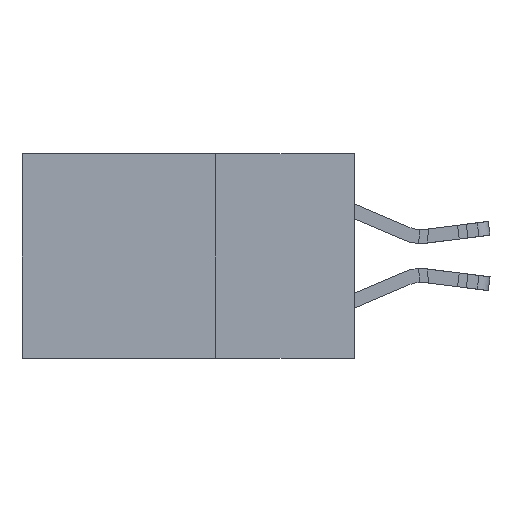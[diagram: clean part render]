
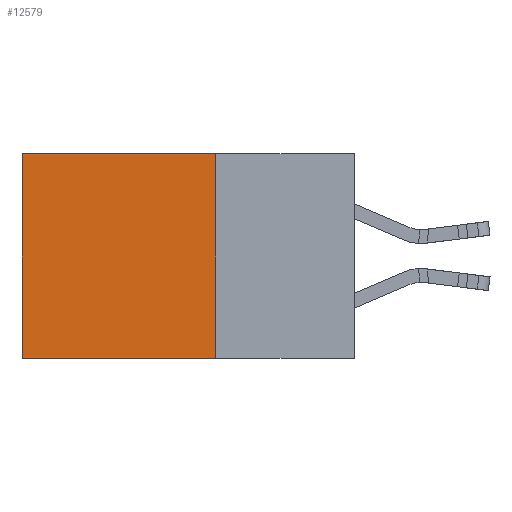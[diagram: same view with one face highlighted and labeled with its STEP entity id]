
A CAD part, left-side view. The second image highlights one B-rep face of the part: STEP entity #12579.
In plain terms, the highlighted planar face has unit normal (-1, 0, 0).
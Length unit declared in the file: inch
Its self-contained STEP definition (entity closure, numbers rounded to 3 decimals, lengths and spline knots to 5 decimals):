
#718 = VERTEX_POINT ( 'NONE', #25084 ) ;
#1443 = VECTOR ( 'NONE', #6467, 39.37008 ) ;
#3622 = EDGE_LOOP ( 'NONE', ( #19263, #14002, #20870, #13499 ) ) ;
#3845 = VERTEX_POINT ( 'NONE', #14104 ) ;
#5294 = EDGE_CURVE ( 'NONE', #3845, #718, #21139, .T. ) ;
#5967 = CARTESIAN_POINT ( 'NONE',  ( 0.2615, 0.25, 0. ) ) ;
#6199 = VECTOR ( 'NONE', #9591, 39.37008 ) ;
#6421 = CARTESIAN_POINT ( 'NONE',  ( 0.2615, 0.25, -0.37 ) ) ;
#6467 = DIRECTION ( 'NONE',  ( 0., 0., -1. ) ) ;
#7890 = PLANE ( 'NONE',  #24392 ) ;
#7988 = DIRECTION ( 'NONE',  ( 0., 1., 0. ) ) ;
#9591 = DIRECTION ( 'NONE',  ( 0., 1., 0. ) ) ;
#9822 = CARTESIAN_POINT ( 'NONE',  ( 0.2615, 0.25, -0.37 ) ) ;
#9906 = DIRECTION ( 'NONE',  ( 0., 0., -1. ) ) ;
#10601 = VECTOR ( 'NONE', #24249, 39.37008 ) ;
#10788 = EDGE_CURVE ( 'NONE', #19904, #14408, #12145, .T. ) ;
#11529 = LINE ( 'NONE', #23343, #6199 ) ;
#12145 = LINE ( 'NONE', #22352, #1443 ) ;
#12579 = ADVANCED_FACE ( 'NONE', ( #23174 ), #7890, .F. ) ;
#13499 = ORIENTED_EDGE ( 'NONE', *, *, #24561, .T. ) ;
#13743 = LINE ( 'NONE', #5967, #14381 ) ;
#14002 = ORIENTED_EDGE ( 'NONE', *, *, #17277, .F. ) ;
#14104 = CARTESIAN_POINT ( 'NONE',  ( 0.2615, 0.25, 0. ) ) ;
#14381 = VECTOR ( 'NONE', #7988, 39.37008 ) ;
#14408 = VERTEX_POINT ( 'NONE', #22714 ) ;
#17277 = EDGE_CURVE ( 'NONE', #718, #14408, #11529, .T. ) ;
#19263 = ORIENTED_EDGE ( 'NONE', *, *, #10788, .T. ) ;
#19385 = CARTESIAN_POINT ( 'NONE',  ( 0.2615, 0.6, 0. ) ) ;
#19904 = VERTEX_POINT ( 'NONE', #19385 ) ;
#20870 = ORIENTED_EDGE ( 'NONE', *, *, #5294, .F. ) ;
#21139 = LINE ( 'NONE', #6421, #10601 ) ;
#21773 = DIRECTION ( 'NONE',  ( 1., 0., 0. ) ) ;
#22352 = CARTESIAN_POINT ( 'NONE',  ( 0.2615, 0.6, -0.37 ) ) ;
#22714 = CARTESIAN_POINT ( 'NONE',  ( 0.2615, 0.6, -0.37 ) ) ;
#23174 = FACE_OUTER_BOUND ( 'NONE', #3622, .T. ) ;
#23343 = CARTESIAN_POINT ( 'NONE',  ( 0.2615, 0.25, -0.37 ) ) ;
#24249 = DIRECTION ( 'NONE',  ( 0., 0., -1. ) ) ;
#24392 = AXIS2_PLACEMENT_3D ( 'NONE', #9822, #21773, #9906 ) ;
#24561 = EDGE_CURVE ( 'NONE', #3845, #19904, #13743, .T. ) ;
#25084 = CARTESIAN_POINT ( 'NONE',  ( 0.2615, 0.25, -0.37 ) ) ;
